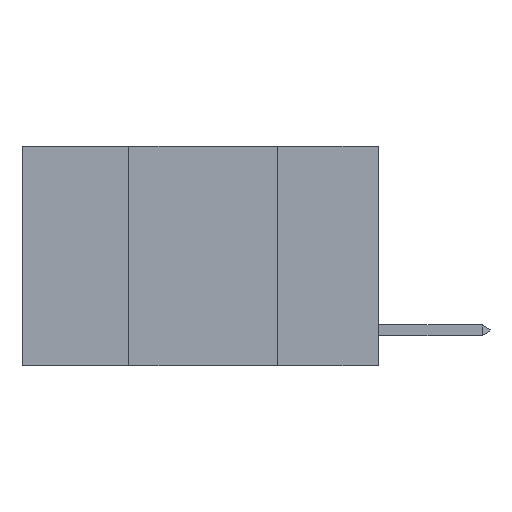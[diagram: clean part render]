
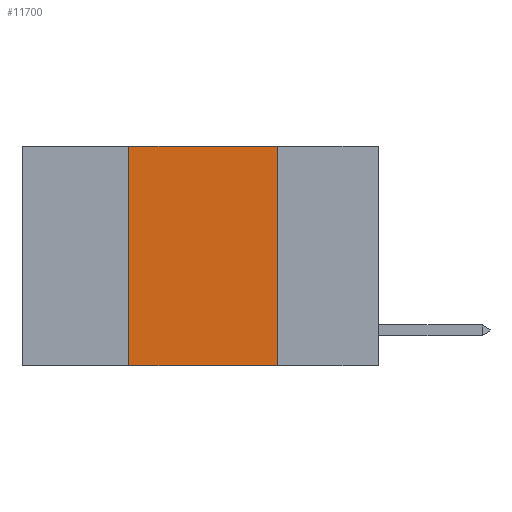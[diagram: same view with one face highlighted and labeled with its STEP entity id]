
A CAD part, left-side view. The second image highlights one B-rep face of the part: STEP entity #11700.
In plain terms, the highlighted planar face has unit normal (-1, 0, 0).
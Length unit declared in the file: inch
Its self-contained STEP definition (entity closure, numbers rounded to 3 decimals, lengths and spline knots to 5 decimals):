
#709 = CARTESIAN_POINT ( 'NONE',  ( 0., 0.6, -0.37 ) ) ;
#730 = CARTESIAN_POINT ( 'NONE',  ( 0., 0.6, 0. ) ) ;
#948 = DIRECTION ( 'NONE',  ( 1., 0., 0. ) ) ;
#1183 = VERTEX_POINT ( 'NONE', #2853 ) ;
#1375 = ORIENTED_EDGE ( 'NONE', *, *, #2864, .T. ) ;
#1723 = EDGE_CURVE ( 'NONE', #1183, #9065, #8136, .T. ) ;
#1778 = CARTESIAN_POINT ( 'NONE',  ( 0., 0.17, -0.37 ) ) ;
#1858 = EDGE_LOOP ( 'NONE', ( #13494, #12608, #8077, #1375 ) ) ;
#2634 = VERTEX_POINT ( 'NONE', #13417 ) ;
#2853 = CARTESIAN_POINT ( 'NONE',  ( 0., 0.42, -0.37 ) ) ;
#2864 = EDGE_CURVE ( 'NONE', #1183, #7945, #5848, .T. ) ;
#3029 = LINE ( 'NONE', #8932, #6243 ) ;
#3254 = DIRECTION ( 'NONE',  ( 0., -1., 0. ) ) ;
#3595 = VECTOR ( 'NONE', #3254, 39.37008 ) ;
#3730 = DIRECTION ( 'NONE',  ( 0., 0., 1. ) ) ;
#3754 = PLANE ( 'NONE',  #12182 ) ;
#4261 = VECTOR ( 'NONE', #3730, 39.37008 ) ;
#4507 = VECTOR ( 'NONE', #4612, 39.37008 ) ;
#4612 = DIRECTION ( 'NONE',  ( 0., 0., -1. ) ) ;
#5848 = LINE ( 'NONE', #709, #3595 ) ;
#6243 = VECTOR ( 'NONE', #8326, 39.37008 ) ;
#6460 = LINE ( 'NONE', #10797, #4507 ) ;
#7945 = VERTEX_POINT ( 'NONE', #1778 ) ;
#8077 = ORIENTED_EDGE ( 'NONE', *, *, #1723, .F. ) ;
#8136 = LINE ( 'NONE', #8207, #4261 ) ;
#8207 = CARTESIAN_POINT ( 'NONE',  ( 0., 0.42, 0. ) ) ;
#8326 = DIRECTION ( 'NONE',  ( 0., -1., 0. ) ) ;
#8364 = CARTESIAN_POINT ( 'NONE',  ( 0., 0.42, 0. ) ) ;
#8932 = CARTESIAN_POINT ( 'NONE',  ( 0., 0.6, 0. ) ) ;
#9065 = VERTEX_POINT ( 'NONE', #8364 ) ;
#10797 = CARTESIAN_POINT ( 'NONE',  ( 0., 0.17, 0. ) ) ;
#11154 = EDGE_CURVE ( 'NONE', #9065, #2634, #3029, .T. ) ;
#11377 = FACE_OUTER_BOUND ( 'NONE', #1858, .T. ) ;
#11700 = ADVANCED_FACE ( 'NONE', ( #11377 ), #3754, .F. ) ;
#12182 = AXIS2_PLACEMENT_3D ( 'NONE', #730, #948, #12208 ) ;
#12208 = DIRECTION ( 'NONE',  ( 0., 0., -1. ) ) ;
#12492 = EDGE_CURVE ( 'NONE', #2634, #7945, #6460, .T. ) ;
#12608 = ORIENTED_EDGE ( 'NONE', *, *, #11154, .F. ) ;
#13417 = CARTESIAN_POINT ( 'NONE',  ( 0., 0.17, 0. ) ) ;
#13494 = ORIENTED_EDGE ( 'NONE', *, *, #12492, .F. ) ;
